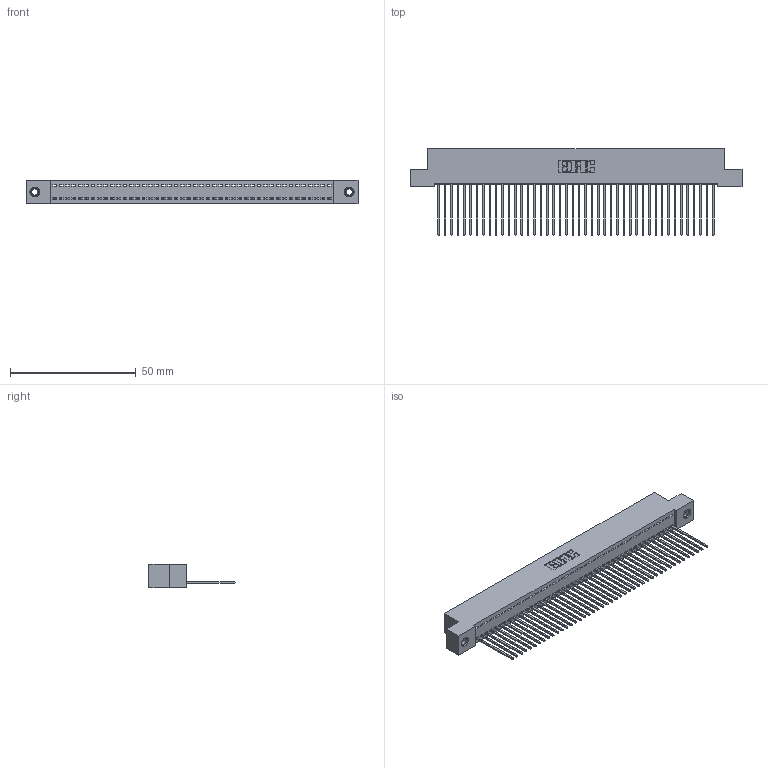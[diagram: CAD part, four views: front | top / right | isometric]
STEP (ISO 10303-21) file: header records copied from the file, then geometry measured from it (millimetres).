
FILE_DESCRIPTION (( 'STEP AP203' ), '1' );
FILE_NAME ('392-044-541-107.STEP', '2018-08-16T15:11:52', ( '' ), ( '' ), 'SwSTEP 2.0', 'SolidWorks 2016', '' );
FILE_SCHEMA (( 'CONFIG_CONTROL_DESIGN' ));
Length unit declared in the file: inch
Products named in the file (4): 345-292-001_345-293-141; 345-250-001_345-250-005-103; 392-044-541-107; 342 Part_TI
Assembly tree (47 placements, depth 2):
  392-044-541-107
    342 Part_TI
    345-292-001_345-293-141  x44
    345-250-001_345-250-005-103  x2
Bounding box: 132.08 x 34.3 x 9.4 mm (x, y, z)
Volume: 11720.7 mm3; surface area: 18106.4 mm2
Topology: 47 solids, 47 shells, 2722 faces, 8179 edges, 5386 vertices
Faces by surface type: plane 1946, cylinder 760, cone 12, torus 4
Entity records: 27712 total; most frequent: CARTESIAN_POINT 4761, ORIENTED_EDGE 4734, DIRECTION 4045, EDGE_CURVE 2367, VECTOR 2219, LINE 2219, VERTEX_POINT 1572, AXIS2_PLACEMENT_3D 913
